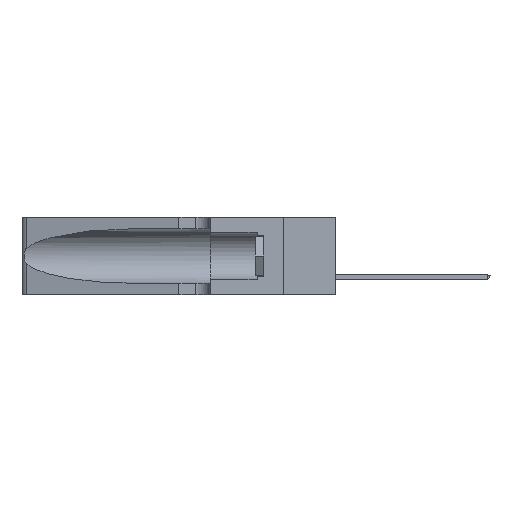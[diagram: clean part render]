
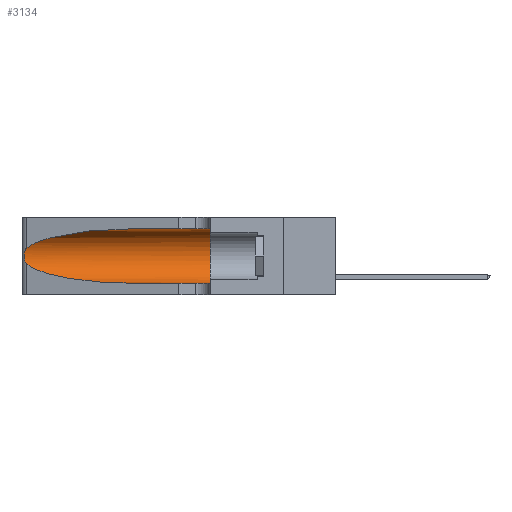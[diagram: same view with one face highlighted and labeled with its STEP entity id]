
A CAD part, left-side view. The second image highlights one B-rep face of the part: STEP entity #3134.
In plain terms, the highlighted cylindrical face has radius 3.308 mm (diameter 6.617 mm), a partial arc.
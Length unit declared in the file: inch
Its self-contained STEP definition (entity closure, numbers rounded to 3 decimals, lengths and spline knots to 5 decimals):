
#1297 = CARTESIAN_POINT ( 'NONE',  ( 0.1305, 1.61858, 0.31525 ) ) ;
#1604 = VERTEX_POINT ( 'NONE', #17282 ) ;
#2217 =( BOUNDED_CURVE ( )  B_SPLINE_CURVE ( 3, ( #10485, #16376, #6457, #19995 ),
 .UNSPECIFIED., .F., .F. ) 
 B_SPLINE_CURVE_WITH_KNOTS ( ( 4, 4 ),
 ( 3.44316, 4.71239 ),
 .UNSPECIFIED. ) 
 CURVE ( )  GEOMETRIC_REPRESENTATION_ITEM ( )  RATIONAL_B_SPLINE_CURVE ( ( 1., 0.87, 0.87, 1. ) ) 
 REPRESENTATION_ITEM ( '' )  );
#2927 = CARTESIAN_POINT ( 'NONE',  ( 0.25639, 1.23184, 0.21858 ) ) ;
#3134 = ADVANCED_FACE ( 'NONE', ( #13003 ), #23497, .F. ) ;
#4003 = LINE ( 'NONE', #7963, #6069 ) ;
#4324 = EDGE_CURVE ( 'NONE', #12317, #1604, #18973, .T. ) ;
#4580 = DIRECTION ( 'NONE',  ( 0., 1., 0. ) ) ;
#4716 = CARTESIAN_POINT ( 'NONE',  ( 0.25555, 1.22993, 0.14849 ) ) ;
#4862 = AXIS2_PLACEMENT_3D ( 'NONE', #16159, #4580, #23603 ) ;
#4879 = CARTESIAN_POINT ( 'NONE',  ( 0.25854, 1.2359, 0.20912 ) ) ;
#5133 = DIRECTION ( 'NONE',  ( 0., -1., 0. ) ) ;
#6069 = VECTOR ( 'NONE', #19684, 39.37008 ) ;
#6094 = VERTEX_POINT ( 'NONE', #11740 ) ;
#6418 = ORIENTED_EDGE ( 'NONE', *, *, #17620, .F. ) ;
#6457 = CARTESIAN_POINT ( 'NONE',  ( 0.18966, 0.96281, 0.05475 ) ) ;
#6798 = CARTESIAN_POINT ( 'NONE',  ( 0.25487, 1.22718, 0.14631 ) ) ;
#7963 = CARTESIAN_POINT ( 'NONE',  ( 0.1305, 1.61858, 0.05475 ) ) ;
#8592 = CARTESIAN_POINT ( 'NONE',  ( 0.25487, 1.22718, 0.22369 ) ) ;
#8950 = ORIENTED_EDGE ( 'NONE', *, *, #15496, .T. ) ;
#9038 = CARTESIAN_POINT ( 'NONE',  ( 0.25487, 1.22718, 0.22369 ) ) ;
#9402 = ORIENTED_EDGE ( 'NONE', *, *, #4324, .F. ) ;
#10485 = CARTESIAN_POINT ( 'NONE',  ( 0.25487, 1.22718, 0.14631 ) ) ;
#10564 = CARTESIAN_POINT ( 'NONE',  ( 0.25856, 1.23593, 0.16098 ) ) ;
#10571 = CARTESIAN_POINT ( 'NONE',  ( 0.1305, 0.35, 0.05475 ) ) ;
#10652 = CARTESIAN_POINT ( 'NONE',  ( 0.25555, 1.22994, 0.2215 ) ) ;
#11030 = ORIENTED_EDGE ( 'NONE', *, *, #21352, .T. ) ;
#11740 = CARTESIAN_POINT ( 'NONE',  ( 0.1305, 0.72297, 0.05475 ) ) ;
#12116 = EDGE_CURVE ( 'NONE', #6094, #17249, #4003, .T. ) ;
#12317 = VERTEX_POINT ( 'NONE', #18159 ) ;
#12419 = CARTESIAN_POINT ( 'NONE',  ( 0.26075, 1.23896, 0.19203 ) ) ;
#12655 = VECTOR ( 'NONE', #17988, 39.37008 ) ;
#13002 = EDGE_CURVE ( 'NONE', #12317, #14600, #24908, .T. ) ;
#13003 = FACE_OUTER_BOUND ( 'NONE', #17856, .T. ) ;
#13452 = ORIENTED_EDGE ( 'NONE', *, *, #13002, .T. ) ;
#13942 = CARTESIAN_POINT ( 'NONE',  ( 0.25487, 1.22718, 0.22369 ) ) ;
#14600 = VERTEX_POINT ( 'NONE', #13942 ) ;
#14789 = CARTESIAN_POINT ( 'NONE',  ( 0.1305, 1.61858, 0.185 ) ) ;
#15496 = EDGE_CURVE ( 'NONE', #22400, #6094, #2217, .T. ) ;
#16159 = CARTESIAN_POINT ( 'NONE',  ( 0.1305, 0.35, 0.185 ) ) ;
#16376 = CARTESIAN_POINT ( 'NONE',  ( 0.2373, 1.15595, 0.08982 ) ) ;
#16454 = CARTESIAN_POINT ( 'NONE',  ( 0.25787, 1.23484, 0.2124 ) ) ;
#17249 = VERTEX_POINT ( 'NONE', #10571 ) ;
#17282 = CARTESIAN_POINT ( 'NONE',  ( 0.1305, 0.35, 0.31525 ) ) ;
#17620 = EDGE_CURVE ( 'NONE', #1604, #17249, #19202, .T. ) ;
#17856 = EDGE_LOOP ( 'NONE', ( #13452, #11030, #8950, #23088, #6418, #9402 ) ) ;
#17988 = DIRECTION ( 'NONE',  ( 0., -1., 0. ) ) ;
#18159 = CARTESIAN_POINT ( 'NONE',  ( 0.1305, 0.72297, 0.31525 ) ) ;
#18369 = CARTESIAN_POINT ( 'NONE',  ( 0.25639, 1.23186, 0.15144 ) ) ;
#18643 = CARTESIAN_POINT ( 'NONE',  ( 0.1305, 0.72297, 0.31525 ) ) ;
#18973 = LINE ( 'NONE', #1297, #12655 ) ;
#19202 = CIRCLE ( 'NONE', #4862, 0.13025 ) ;
#19684 = DIRECTION ( 'NONE',  ( 0., -1., 0. ) ) ;
#19995 = CARTESIAN_POINT ( 'NONE',  ( 0.1305, 0.72297, 0.05475 ) ) ;
#20328 = CARTESIAN_POINT ( 'NONE',  ( 0.26017, 1.23833, 0.17102 ) ) ;
#20683 = CARTESIAN_POINT ( 'NONE',  ( 0.2373, 1.15595, 0.28018 ) ) ;
#21352 = EDGE_CURVE ( 'NONE', #14600, #22400, #24586, .T. ) ;
#22077 = CARTESIAN_POINT ( 'NONE',  ( 0.26018, 1.23835, 0.19895 ) ) ;
#22400 = VERTEX_POINT ( 'NONE', #23129 ) ;
#23088 = ORIENTED_EDGE ( 'NONE', *, *, #12116, .T. ) ;
#23129 = CARTESIAN_POINT ( 'NONE',  ( 0.25487, 1.22718, 0.14631 ) ) ;
#23239 = DIRECTION ( 'NONE',  ( 0., 0., -1. ) ) ;
#23497 = CYLINDRICAL_SURFACE ( 'NONE', #24597, 0.13025 ) ;
#23603 = DIRECTION ( 'NONE',  ( 0., 0., 1. ) ) ;
#23977 = CARTESIAN_POINT ( 'NONE',  ( 0.25789, 1.23486, 0.15765 ) ) ;
#24058 = CARTESIAN_POINT ( 'NONE',  ( 0.26075, 1.23896, 0.178 ) ) ;
#24151 = CARTESIAN_POINT ( 'NONE',  ( 0.18966, 0.96281, 0.31525 ) ) ;
#24586 = B_SPLINE_CURVE_WITH_KNOTS ( 'NONE', 3,
 ( #8592, #10652, #2927, #16454, #4879, #22077, #12419, #24058, #20328, #10564, #23977, #18369, #4716, #6798 ),
 .UNSPECIFIED., .F., .F.,
 ( 4, 2, 2, 2, 2, 2, 4 ),
 ( 0., 0.00027, 0.00053, 0.00107, 0.0016, 0.00187, 0.00214 ),
 .UNSPECIFIED. ) ;
#24597 = AXIS2_PLACEMENT_3D ( 'NONE', #14789, #5133, #23239 ) ;
#24908 =( BOUNDED_CURVE ( )  B_SPLINE_CURVE ( 3, ( #18643, #24151, #20683, #9038 ),
 .UNSPECIFIED., .F., .F. ) 
 B_SPLINE_CURVE_WITH_KNOTS ( ( 4, 4 ),
 ( 1.5708, 2.84003 ),
 .UNSPECIFIED. ) 
 CURVE ( )  GEOMETRIC_REPRESENTATION_ITEM ( )  RATIONAL_B_SPLINE_CURVE ( ( 1., 0.87, 0.87, 1. ) ) 
 REPRESENTATION_ITEM ( '' )  );
